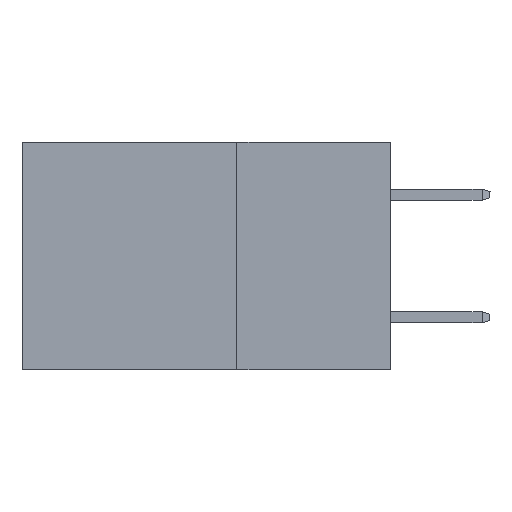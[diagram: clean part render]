
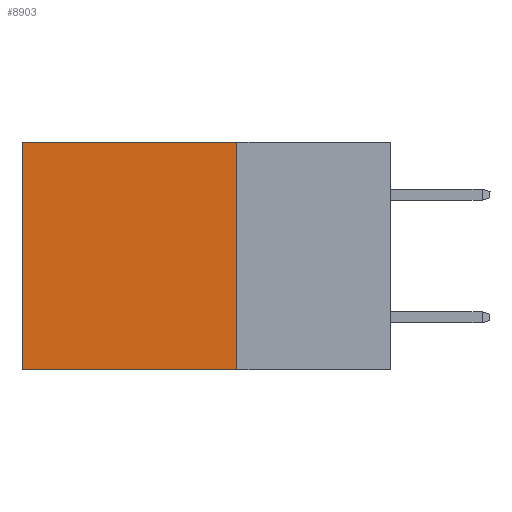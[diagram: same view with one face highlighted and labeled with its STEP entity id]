
A CAD part, left-side view. The second image highlights one B-rep face of the part: STEP entity #8903.
In plain terms, the highlighted planar face has unit normal (-1, 0, 0).
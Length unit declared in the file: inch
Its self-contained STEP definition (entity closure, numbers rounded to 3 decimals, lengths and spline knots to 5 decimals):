
#457 = CARTESIAN_POINT ( 'NONE',  ( 0.2875, 0.25, 0. ) ) ;
#710 = VERTEX_POINT ( 'NONE', #6699 ) ;
#723 = LINE ( 'NONE', #457, #2542 ) ;
#1027 = VERTEX_POINT ( 'NONE', #1935 ) ;
#1529 = CARTESIAN_POINT ( 'NONE',  ( 0.2875, 0.25, -0.37 ) ) ;
#1935 = CARTESIAN_POINT ( 'NONE',  ( 0.2875, 0.25, -0.37 ) ) ;
#2141 = FACE_OUTER_BOUND ( 'NONE', #2844, .T. ) ;
#2267 = CARTESIAN_POINT ( 'NONE',  ( 0.2875, 0.6, 0. ) ) ;
#2542 = VECTOR ( 'NONE', #9243, 39.37008 ) ;
#2620 = VECTOR ( 'NONE', #10305, 39.37008 ) ;
#2844 = EDGE_LOOP ( 'NONE', ( #3185, #9472, #6445, #8497 ) ) ;
#3185 = ORIENTED_EDGE ( 'NONE', *, *, #3369, .T. ) ;
#3369 = EDGE_CURVE ( 'NONE', #10979, #710, #9350, .T. ) ;
#3421 = EDGE_CURVE ( 'NONE', #11114, #1027, #723, .T. ) ;
#3496 = CARTESIAN_POINT ( 'NONE',  ( 0.2875, 0.25, 0. ) ) ;
#4024 = CARTESIAN_POINT ( 'NONE',  ( 0.2875, 0.25, 0. ) ) ;
#4414 = EDGE_CURVE ( 'NONE', #1027, #710, #8782, .T. ) ;
#4697 = VECTOR ( 'NONE', #9698, 39.37008 ) ;
#5321 = AXIS2_PLACEMENT_3D ( 'NONE', #4024, #5829, #8600 ) ;
#5829 = DIRECTION ( 'NONE',  ( 1., 0., 0. ) ) ;
#5856 = EDGE_CURVE ( 'NONE', #11114, #10979, #7101, .T. ) ;
#6445 = ORIENTED_EDGE ( 'NONE', *, *, #3421, .F. ) ;
#6699 = CARTESIAN_POINT ( 'NONE',  ( 0.2875, 0.6, -0.37 ) ) ;
#7101 = LINE ( 'NONE', #9512, #2620 ) ;
#8365 = PLANE ( 'NONE',  #5321 ) ;
#8497 = ORIENTED_EDGE ( 'NONE', *, *, #5856, .T. ) ;
#8600 = DIRECTION ( 'NONE',  ( 0., 0., -1. ) ) ;
#8782 = LINE ( 'NONE', #1529, #10138 ) ;
#8903 = ADVANCED_FACE ( 'NONE', ( #2141 ), #8365, .F. ) ;
#8980 = DIRECTION ( 'NONE',  ( 0., 1., 0. ) ) ;
#9243 = DIRECTION ( 'NONE',  ( 0., 0., -1. ) ) ;
#9350 = LINE ( 'NONE', #10542, #4697 ) ;
#9472 = ORIENTED_EDGE ( 'NONE', *, *, #4414, .F. ) ;
#9512 = CARTESIAN_POINT ( 'NONE',  ( 0.2875, 0.25, 0. ) ) ;
#9698 = DIRECTION ( 'NONE',  ( 0., 0., -1. ) ) ;
#10138 = VECTOR ( 'NONE', #8980, 39.37008 ) ;
#10305 = DIRECTION ( 'NONE',  ( 0., 1., 0. ) ) ;
#10542 = CARTESIAN_POINT ( 'NONE',  ( 0.2875, 0.6, 0. ) ) ;
#10979 = VERTEX_POINT ( 'NONE', #2267 ) ;
#11114 = VERTEX_POINT ( 'NONE', #3496 ) ;
